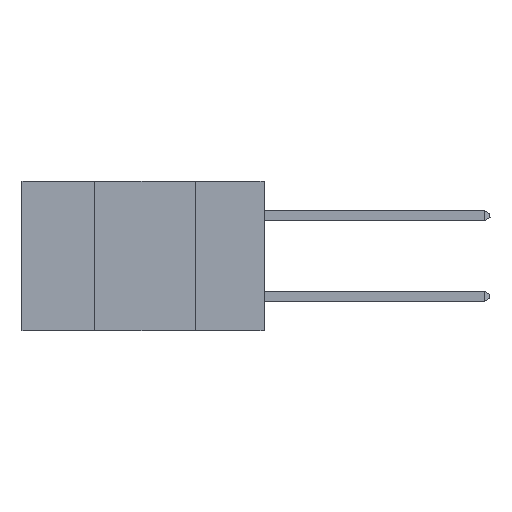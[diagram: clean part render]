
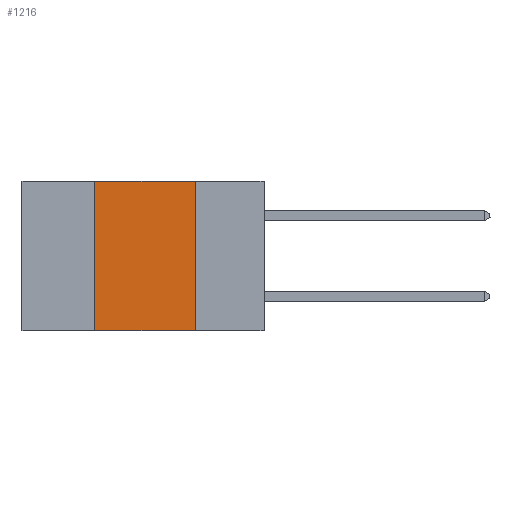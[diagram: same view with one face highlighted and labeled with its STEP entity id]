
A CAD part, left-side view. The second image highlights one B-rep face of the part: STEP entity #1216.
In plain terms, the highlighted planar face has unit normal (-1, 0, 0).
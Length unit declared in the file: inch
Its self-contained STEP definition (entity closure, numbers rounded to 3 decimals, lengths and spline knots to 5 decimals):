
#105 = ORIENTED_EDGE ( 'NONE', *, *, #10980, .T. ) ;
#471 = ORIENTED_EDGE ( 'NONE', *, *, #757, .F. ) ;
#757 = EDGE_CURVE ( 'NONE', #2833, #3856, #8639, .T. ) ;
#948 = VERTEX_POINT ( 'NONE', #2108 ) ;
#970 = EDGE_LOOP ( 'NONE', ( #471, #6178, #6193, #105 ) ) ;
#1121 = AXIS2_PLACEMENT_3D ( 'NONE', #10266, #8633, #5102 ) ;
#1216 = ADVANCED_FACE ( 'NONE', ( #1233 ), #4108, .F. ) ;
#1233 = FACE_OUTER_BOUND ( 'NONE', #970, .T. ) ;
#1879 = DIRECTION ( 'NONE',  ( 0., 0., 1. ) ) ;
#2108 = CARTESIAN_POINT ( 'NONE',  ( 0., 0.42, -0.37 ) ) ;
#2833 = VERTEX_POINT ( 'NONE', #6775 ) ;
#2868 = CARTESIAN_POINT ( 'NONE',  ( 0., 0.6, 0. ) ) ;
#3508 = CARTESIAN_POINT ( 'NONE',  ( 0., 0.42, 0. ) ) ;
#3856 = VERTEX_POINT ( 'NONE', #9556 ) ;
#3863 = CARTESIAN_POINT ( 'NONE',  ( 0., 0.42, 0. ) ) ;
#3959 = LINE ( 'NONE', #3508, #10274 ) ;
#4108 = PLANE ( 'NONE',  #1121 ) ;
#4658 = DIRECTION ( 'NONE',  ( 0., 0., -1. ) ) ;
#5102 = DIRECTION ( 'NONE',  ( 0., 0., -1. ) ) ;
#5199 = VECTOR ( 'NONE', #4658, 39.37008 ) ;
#5791 = VECTOR ( 'NONE', #7167, 39.37008 ) ;
#6178 = ORIENTED_EDGE ( 'NONE', *, *, #8664, .F. ) ;
#6193 = ORIENTED_EDGE ( 'NONE', *, *, #10334, .F. ) ;
#6275 = LINE ( 'NONE', #8533, #6406 ) ;
#6406 = VECTOR ( 'NONE', #9442, 39.37008 ) ;
#6601 = CARTESIAN_POINT ( 'NONE',  ( 0., 0.17, 0. ) ) ;
#6775 = CARTESIAN_POINT ( 'NONE',  ( 0., 0.17, 0. ) ) ;
#7167 = DIRECTION ( 'NONE',  ( 0., -1., 0. ) ) ;
#8031 = VERTEX_POINT ( 'NONE', #3863 ) ;
#8533 = CARTESIAN_POINT ( 'NONE',  ( 0., 0.6, -0.37 ) ) ;
#8633 = DIRECTION ( 'NONE',  ( 1., 0., 0. ) ) ;
#8639 = LINE ( 'NONE', #6601, #5199 ) ;
#8664 = EDGE_CURVE ( 'NONE', #8031, #2833, #9773, .T. ) ;
#9442 = DIRECTION ( 'NONE',  ( 0., -1., 0. ) ) ;
#9556 = CARTESIAN_POINT ( 'NONE',  ( 0., 0.17, -0.37 ) ) ;
#9773 = LINE ( 'NONE', #2868, #5791 ) ;
#10266 = CARTESIAN_POINT ( 'NONE',  ( 0., 0.6, 0. ) ) ;
#10274 = VECTOR ( 'NONE', #1879, 39.37008 ) ;
#10334 = EDGE_CURVE ( 'NONE', #948, #8031, #3959, .T. ) ;
#10980 = EDGE_CURVE ( 'NONE', #948, #3856, #6275, .T. ) ;
